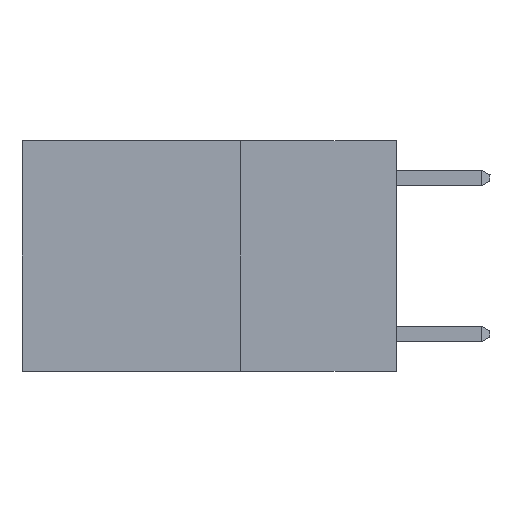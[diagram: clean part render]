
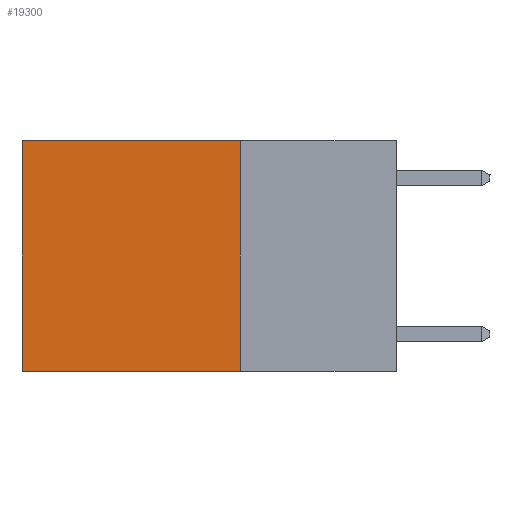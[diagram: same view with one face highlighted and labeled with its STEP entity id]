
A CAD part, left-side view. The second image highlights one B-rep face of the part: STEP entity #19300.
In plain terms, the highlighted planar face has unit normal (-1, 0, 0).
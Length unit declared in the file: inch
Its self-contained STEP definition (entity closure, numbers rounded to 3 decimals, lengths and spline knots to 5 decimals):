
#266 = CARTESIAN_POINT ( 'NONE',  ( 0.2625, 0.6, 0. ) ) ;
#1490 = CARTESIAN_POINT ( 'NONE',  ( 0.2625, 0.25, -0.37 ) ) ;
#1760 = DIRECTION ( 'NONE',  ( 0., 0., -1. ) ) ;
#2251 = VECTOR ( 'NONE', #10464, 39.37008 ) ;
#2266 = PLANE ( 'NONE',  #4063 ) ;
#4063 = AXIS2_PLACEMENT_3D ( 'NONE', #7772, #21516, #9126 ) ;
#4379 = CARTESIAN_POINT ( 'NONE',  ( 0.2625, 0.6, 0. ) ) ;
#4727 = CARTESIAN_POINT ( 'NONE',  ( 0.2625, 0.25, 0. ) ) ;
#5063 = LINE ( 'NONE', #10240, #2251 ) ;
#5348 = VERTEX_POINT ( 'NONE', #4379 ) ;
#6282 = LINE ( 'NONE', #4727, #20725 ) ;
#7443 = CARTESIAN_POINT ( 'NONE',  ( 0.2625, 0.25, 0. ) ) ;
#7547 = EDGE_CURVE ( 'NONE', #19176, #8070, #22228, .T. ) ;
#7772 = CARTESIAN_POINT ( 'NONE',  ( 0.2625, 0.25, 0. ) ) ;
#8070 = VERTEX_POINT ( 'NONE', #13247 ) ;
#9126 = DIRECTION ( 'NONE',  ( 0., 0., -1. ) ) ;
#9943 = DIRECTION ( 'NONE',  ( 0., 1., 0. ) ) ;
#10240 = CARTESIAN_POINT ( 'NONE',  ( 0.2625, 0.25, 0. ) ) ;
#10464 = DIRECTION ( 'NONE',  ( 0., 1., 0. ) ) ;
#11210 = EDGE_CURVE ( 'NONE', #5348, #8070, #17292, .T. ) ;
#12815 = ORIENTED_EDGE ( 'NONE', *, *, #18015, .F. ) ;
#13247 = CARTESIAN_POINT ( 'NONE',  ( 0.2625, 0.6, -0.37 ) ) ;
#13310 = DIRECTION ( 'NONE',  ( 0., 0., -1. ) ) ;
#13620 = ORIENTED_EDGE ( 'NONE', *, *, #7547, .F. ) ;
#14433 = CARTESIAN_POINT ( 'NONE',  ( 0.2625, 0.25, -0.37 ) ) ;
#14886 = VECTOR ( 'NONE', #1760, 39.37008 ) ;
#15130 = VECTOR ( 'NONE', #9943, 39.37008 ) ;
#15527 = EDGE_LOOP ( 'NONE', ( #18480, #13620, #12815, #18024 ) ) ;
#17292 = LINE ( 'NONE', #266, #14886 ) ;
#17681 = FACE_OUTER_BOUND ( 'NONE', #15527, .T. ) ;
#18015 = EDGE_CURVE ( 'NONE', #19305, #19176, #6282, .T. ) ;
#18024 = ORIENTED_EDGE ( 'NONE', *, *, #21013, .T. ) ;
#18480 = ORIENTED_EDGE ( 'NONE', *, *, #11210, .T. ) ;
#19176 = VERTEX_POINT ( 'NONE', #14433 ) ;
#19300 = ADVANCED_FACE ( 'NONE', ( #17681 ), #2266, .F. ) ;
#19305 = VERTEX_POINT ( 'NONE', #7443 ) ;
#20725 = VECTOR ( 'NONE', #13310, 39.37008 ) ;
#21013 = EDGE_CURVE ( 'NONE', #19305, #5348, #5063, .T. ) ;
#21516 = DIRECTION ( 'NONE',  ( 1., 0., 0. ) ) ;
#22228 = LINE ( 'NONE', #1490, #15130 ) ;
